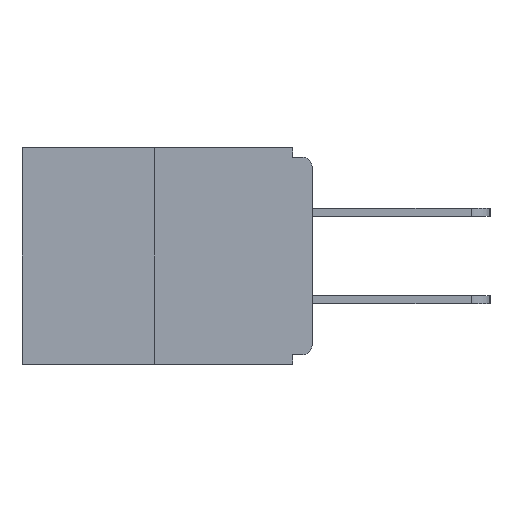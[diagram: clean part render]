
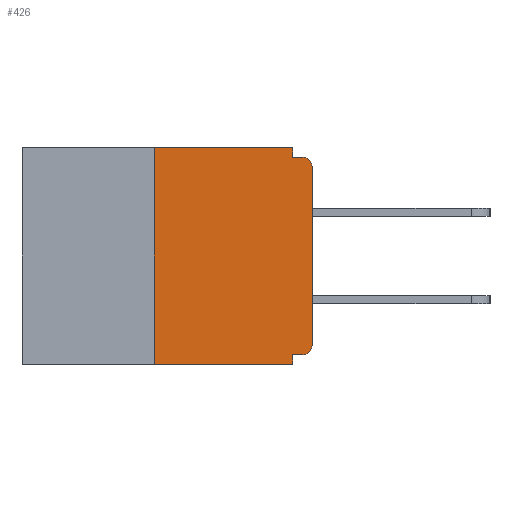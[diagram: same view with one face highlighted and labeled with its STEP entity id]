
A CAD part, left-side view. The second image highlights one B-rep face of the part: STEP entity #426.
In plain terms, the highlighted planar face has unit normal (-1, 0, 0).
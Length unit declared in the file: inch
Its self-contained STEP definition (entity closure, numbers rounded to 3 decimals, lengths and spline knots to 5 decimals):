
#144 = DIRECTION ( 'NONE',  ( 0., 0., -1. ) ) ;
#426 = ADVANCED_FACE ( 'NONE', ( #12371 ), #9006, .F. ) ;
#639 = VECTOR ( 'NONE', #5466, 39.37008 ) ;
#1008 = DIRECTION ( 'NONE',  ( 0., 0., 1. ) ) ;
#1145 = ORIENTED_EDGE ( 'NONE', *, *, #2383, .F. ) ;
#1393 = CARTESIAN_POINT ( 'NONE',  ( 0., 0.031, -0.015 ) ) ;
#1464 = EDGE_CURVE ( 'NONE', #17547, #8553, #13405, .T. ) ;
#1936 = VERTEX_POINT ( 'NONE', #16810 ) ;
#1965 = ORIENTED_EDGE ( 'NONE', *, *, #13270, .F. ) ;
#2339 = DIRECTION ( 'NONE',  ( 0., 0., -1. ) ) ;
#2359 = CARTESIAN_POINT ( 'NONE',  ( 0., 0.031, -0.328 ) ) ;
#2383 = EDGE_CURVE ( 'NONE', #13738, #8089, #3974, .T. ) ;
#2406 = ORIENTED_EDGE ( 'NONE', *, *, #10135, .T. ) ;
#3004 = DIRECTION ( 'NONE',  ( 0., -1., 0. ) ) ;
#3115 = ORIENTED_EDGE ( 'NONE', *, *, #4306, .F. ) ;
#3585 = EDGE_CURVE ( 'NONE', #8089, #17547, #16086, .T. ) ;
#3752 = CARTESIAN_POINT ( 'NONE',  ( 0., 0., 0. ) ) ;
#3837 = DIRECTION ( 'NONE',  ( 0., 0., -1. ) ) ;
#3969 = AXIS2_PLACEMENT_3D ( 'NONE', #11571, #8002, #3837 ) ;
#3974 = LINE ( 'NONE', #8473, #8436 ) ;
#4306 = EDGE_CURVE ( 'NONE', #10031, #16642, #16515, .T. ) ;
#4888 = VERTEX_POINT ( 'NONE', #13526 ) ;
#5181 = VECTOR ( 'NONE', #1008, 39.37008 ) ;
#5466 = DIRECTION ( 'NONE',  ( 0., 0., -1. ) ) ;
#5567 = DIRECTION ( 'NONE',  ( 0., 1., 0. ) ) ;
#5581 = EDGE_CURVE ( 'NONE', #17645, #9464, #13491, .T. ) ;
#6333 = DIRECTION ( 'NONE',  ( 0., -1., 0. ) ) ;
#6357 = CARTESIAN_POINT ( 'NONE',  ( 0., 0.015, -0.03 ) ) ;
#6607 = DIRECTION ( 'NONE',  ( 0., 0., -1. ) ) ;
#6836 = ORIENTED_EDGE ( 'NONE', *, *, #7758, .T. ) ;
#7090 = CARTESIAN_POINT ( 'NONE',  ( 0., 0.031, 0. ) ) ;
#7758 = EDGE_CURVE ( 'NONE', #9464, #4888, #8113, .T. ) ;
#7783 = CIRCLE ( 'NONE', #13509, 0.015 ) ;
#8002 = DIRECTION ( 'NONE',  ( 1., 0., 0. ) ) ;
#8089 = VERTEX_POINT ( 'NONE', #11671 ) ;
#8113 = CIRCLE ( 'NONE', #9224, 0.015 ) ;
#8193 = EDGE_CURVE ( 'NONE', #8553, #4888, #14945, .T. ) ;
#8436 = VECTOR ( 'NONE', #15224, 39.37008 ) ;
#8473 = CARTESIAN_POINT ( 'NONE',  ( 0., 0.25, 0. ) ) ;
#8553 = VERTEX_POINT ( 'NONE', #1393 ) ;
#9006 = PLANE ( 'NONE',  #3969 ) ;
#9224 = AXIS2_PLACEMENT_3D ( 'NONE', #6357, #14400, #2339 ) ;
#9464 = VERTEX_POINT ( 'NONE', #12347 ) ;
#9613 = CARTESIAN_POINT ( 'NONE',  ( 0., 0.031, -0.343 ) ) ;
#9746 = ORIENTED_EDGE ( 'NONE', *, *, #11007, .T. ) ;
#10031 = VERTEX_POINT ( 'NONE', #10787 ) ;
#10135 = EDGE_CURVE ( 'NONE', #13738, #1936, #14449, .T. ) ;
#10787 = CARTESIAN_POINT ( 'NONE',  ( 0., 0.015, -0.328 ) ) ;
#11007 = EDGE_CURVE ( 'NONE', #10031, #17645, #7783, .T. ) ;
#11134 = CARTESIAN_POINT ( 'NONE',  ( 0., 0.25, -0.343 ) ) ;
#11247 = EDGE_LOOP ( 'NONE', ( #15184, #1145, #2406, #1965, #3115, #9746, #12053, #6836, #13328, #13439 ) ) ;
#11571 = CARTESIAN_POINT ( 'NONE',  ( 0., 0.46, 0. ) ) ;
#11635 = VECTOR ( 'NONE', #3004, 39.37008 ) ;
#11671 = CARTESIAN_POINT ( 'NONE',  ( 0., 0.25, 0. ) ) ;
#12002 = CARTESIAN_POINT ( 'NONE',  ( 0., 0.015, -0.313 ) ) ;
#12053 = ORIENTED_EDGE ( 'NONE', *, *, #5581, .T. ) ;
#12319 = CARTESIAN_POINT ( 'NONE',  ( 0., 0., -0.328 ) ) ;
#12347 = CARTESIAN_POINT ( 'NONE',  ( 0., 0., -0.03 ) ) ;
#12371 = FACE_OUTER_BOUND ( 'NONE', #11247, .T. ) ;
#12392 = DIRECTION ( 'NONE',  ( 0., -1., 0. ) ) ;
#12991 = LINE ( 'NONE', #9613, #639 ) ;
#13270 = EDGE_CURVE ( 'NONE', #16642, #1936, #12991, .T. ) ;
#13328 = ORIENTED_EDGE ( 'NONE', *, *, #8193, .F. ) ;
#13405 = LINE ( 'NONE', #7090, #13825 ) ;
#13439 = ORIENTED_EDGE ( 'NONE', *, *, #1464, .F. ) ;
#13491 = LINE ( 'NONE', #3752, #5181 ) ;
#13509 = AXIS2_PLACEMENT_3D ( 'NONE', #12002, #14758, #6607 ) ;
#13526 = CARTESIAN_POINT ( 'NONE',  ( 0., 0.015, -0.015 ) ) ;
#13738 = VERTEX_POINT ( 'NONE', #11134 ) ;
#13825 = VECTOR ( 'NONE', #144, 39.37008 ) ;
#14144 = CARTESIAN_POINT ( 'NONE',  ( 0., 0.031, 0. ) ) ;
#14400 = DIRECTION ( 'NONE',  ( -1., 0., 0. ) ) ;
#14449 = LINE ( 'NONE', #16742, #11635 ) ;
#14486 = CARTESIAN_POINT ( 'NONE',  ( 0., 0., -0.015 ) ) ;
#14610 = CARTESIAN_POINT ( 'NONE',  ( 0., 0., -0.313 ) ) ;
#14758 = DIRECTION ( 'NONE',  ( -1., 0., 0. ) ) ;
#14945 = LINE ( 'NONE', #14486, #16198 ) ;
#15184 = ORIENTED_EDGE ( 'NONE', *, *, #3585, .F. ) ;
#15224 = DIRECTION ( 'NONE',  ( 0., 0., 1. ) ) ;
#15313 = CARTESIAN_POINT ( 'NONE',  ( 0., 0.46, 0. ) ) ;
#16086 = LINE ( 'NONE', #15313, #17600 ) ;
#16198 = VECTOR ( 'NONE', #6333, 39.37008 ) ;
#16515 = LINE ( 'NONE', #12319, #17603 ) ;
#16642 = VERTEX_POINT ( 'NONE', #2359 ) ;
#16742 = CARTESIAN_POINT ( 'NONE',  ( 0., 0.46, -0.343 ) ) ;
#16810 = CARTESIAN_POINT ( 'NONE',  ( 0., 0.031, -0.343 ) ) ;
#17547 = VERTEX_POINT ( 'NONE', #14144 ) ;
#17600 = VECTOR ( 'NONE', #12392, 39.37008 ) ;
#17603 = VECTOR ( 'NONE', #5567, 39.37008 ) ;
#17645 = VERTEX_POINT ( 'NONE', #14610 ) ;
